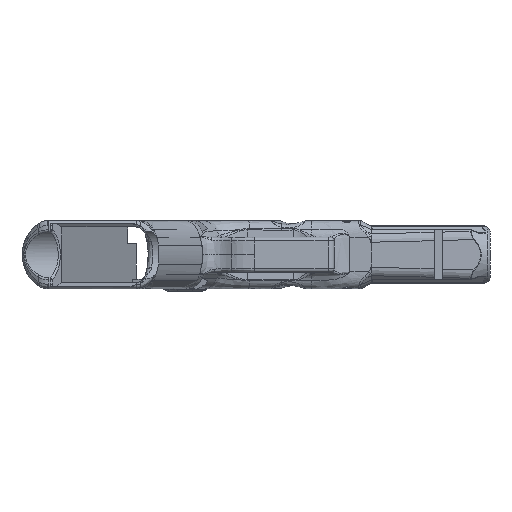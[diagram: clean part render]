
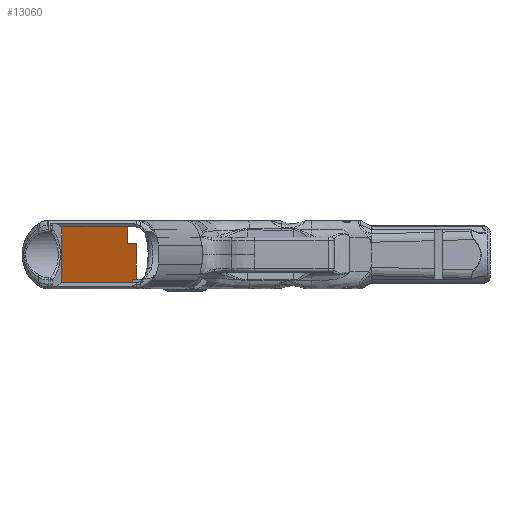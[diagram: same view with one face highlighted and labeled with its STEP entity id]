
A CAD part, front view. The second image highlights one B-rep face of the part: STEP entity #13060.
In plain terms, the highlighted planar face has unit normal (0.951, -0.309, 0).
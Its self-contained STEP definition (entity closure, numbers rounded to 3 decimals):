
#2170=FACE_OUTER_BOUND('',#2909,.T.);
#2909=EDGE_LOOP('',(#11252,#11253,#11254,#11255,#11256,#11257,#11258,#11259,
#11260,#11261));
#3425=LINE('',#27263,#4245);
#3548=LINE('',#31656,#4368);
#3559=LINE('',#32111,#4379);
#3701=LINE('',#44082,#4521);
#3724=LINE('',#45819,#4544);
#3728=LINE('',#46128,#4548);
#3734=LINE('',#46740,#4554);
#3735=LINE('',#46741,#4555);
#4245=VECTOR('',#15296,10.);
#4368=VECTOR('',#15769,10.);
#4379=VECTOR('',#15808,10.);
#4521=VECTOR('',#16450,10.);
#4544=VECTOR('',#16591,10.);
#4548=VECTOR('',#16601,10.);
#4554=VECTOR('',#16637,10.);
#4555=VECTOR('',#16638,10.);
#4784=ELLIPSE('',#13771,1.051,1.);
#4794=ELLIPSE('',#13798,1.051,1.);
#5396=VERTEX_POINT('',#27260);
#5397=VERTEX_POINT('',#27262);
#5549=VERTEX_POINT('',#30602);
#5590=VERTEX_POINT('',#31631);
#5592=VERTEX_POINT('',#31635);
#5600=VERTEX_POINT('',#31654);
#5952=VERTEX_POINT('',#44080);
#5988=VERTEX_POINT('',#45818);
#5995=VERTEX_POINT('',#46125);
#5996=VERTEX_POINT('',#46127);
#6882=EDGE_CURVE('',#5397,#5396,#3425,.T.);
#7122=EDGE_CURVE('',#5549,#5396,#4784,.F.);
#7181=EDGE_CURVE('',#5592,#5590,#4794,.F.);
#7191=EDGE_CURVE('',#5592,#5600,#3548,.T.);
#7221=EDGE_CURVE('',#5590,#5549,#3559,.F.);
#7762=EDGE_CURVE('',#5952,#5600,#3701,.T.);
#7838=EDGE_CURVE('',#5988,#5952,#3724,.T.);
#7848=EDGE_CURVE('',#5995,#5996,#3728,.T.);
#7865=EDGE_CURVE('',#5996,#5988,#3734,.T.);
#7866=EDGE_CURVE('',#5397,#5995,#3735,.T.);
#11252=ORIENTED_EDGE('',*,*,#6882,.T.);
#11253=ORIENTED_EDGE('',*,*,#7122,.F.);
#11254=ORIENTED_EDGE('',*,*,#7221,.F.);
#11255=ORIENTED_EDGE('',*,*,#7181,.F.);
#11256=ORIENTED_EDGE('',*,*,#7191,.T.);
#11257=ORIENTED_EDGE('',*,*,#7762,.F.);
#11258=ORIENTED_EDGE('',*,*,#7838,.F.);
#11259=ORIENTED_EDGE('',*,*,#7865,.F.);
#11260=ORIENTED_EDGE('',*,*,#7848,.F.);
#11261=ORIENTED_EDGE('',*,*,#7866,.F.);
#12442=PLANE('',#14140);
#13060=ADVANCED_FACE('',(#2170),#12442,.F.);
#13771=AXIS2_PLACEMENT_3D('',#30603,#15695,#15696);
#13798=AXIS2_PLACEMENT_3D('',#31637,#15756,#15757);
#14140=AXIS2_PLACEMENT_3D('',#46739,#16635,#16636);
#15296=DIRECTION('',(-0.309,-0.951,0.));
#15695=DIRECTION('center_axis',(-0.951,0.309,0.));
#15696=DIRECTION('ref_axis',(-0.309,-0.951,0.));
#15756=DIRECTION('center_axis',(-0.951,0.309,0.));
#15757=DIRECTION('ref_axis',(-0.309,-0.951,0.));
#15769=DIRECTION('',(0.309,0.951,0.));
#15808=DIRECTION('',(0.,0.,-1.));
#16450=DIRECTION('',(0.,0.,-1.));
#16591=DIRECTION('',(-0.309,-0.951,0.));
#16601=DIRECTION('',(0.309,0.951,0.));
#16635=DIRECTION('center_axis',(-0.951,0.309,0.));
#16636=DIRECTION('ref_axis',(0.,0.,
1.));
#16637=DIRECTION('',(0.,0.,-1.));
#16638=DIRECTION('',(0.,0.,-1.));
#27260=CARTESIAN_POINT('',(2.294,-97.822,11.75));
#27262=CARTESIAN_POINT('',(30.049,-12.4,11.75));
#27263=CARTESIAN_POINT('',(2.312,-97.765,11.75));
#30602=CARTESIAN_POINT('',(2.236,-98.,11.766));
#30603=CARTESIAN_POINT('Origin',(2.294,-97.822,12.75));
#31631=CARTESIAN_POINT('',(2.236,-98.,-11.766));
#31635=CARTESIAN_POINT('',(2.294,-97.822,-11.75));
#31637=CARTESIAN_POINT('Origin',(2.294,-97.822,-12.75));
#31654=CARTESIAN_POINT('',(32.169,-5.875,-11.75));
#31656=CARTESIAN_POINT('',(2.312,-97.765,-11.75));
#32111=CARTESIAN_POINT('',(2.236,-98.,-18.375));
#44080=CARTESIAN_POINT('',(32.169,-5.875,-10.375));
#44082=CARTESIAN_POINT('',(32.169,-5.875,-5.875));
#45818=CARTESIAN_POINT('',(33.591,-1.5,-10.375));
#45819=CARTESIAN_POINT('',(17.241,-51.82,-10.375));
#46125=CARTESIAN_POINT('',(30.049,-12.4,4.75));
#46127=CARTESIAN_POINT('',(33.591,-1.5,4.75));
#46128=CARTESIAN_POINT('',(18.86,-46.836,4.75));
#46739=CARTESIAN_POINT('Origin',(2.312,-97.765,-11.75));
#46740=CARTESIAN_POINT('',(33.591,-1.5,-5.875));
#46741=CARTESIAN_POINT('',(30.049,-12.4,2.982));
